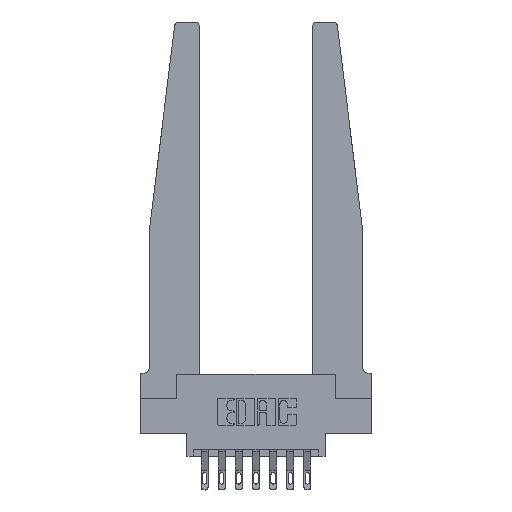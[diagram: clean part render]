
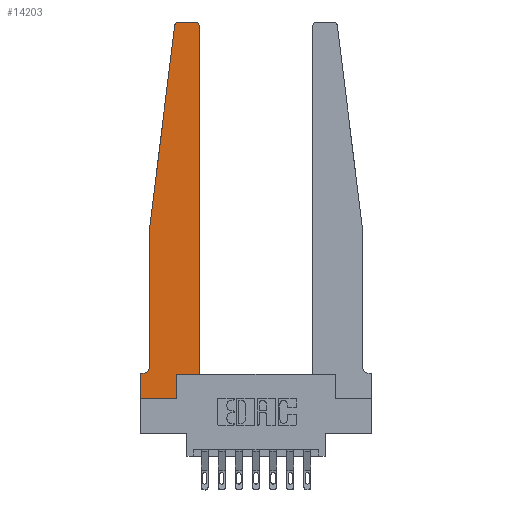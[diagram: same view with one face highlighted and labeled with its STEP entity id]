
A CAD part, top view. The second image highlights one B-rep face of the part: STEP entity #14203.
In plain terms, the highlighted planar face has unit normal (0, 0, 1).
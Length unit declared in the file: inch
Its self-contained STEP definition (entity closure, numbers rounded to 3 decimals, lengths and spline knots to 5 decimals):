
#32 = VECTOR ( 'NONE', #11932, 39.37008 ) ;
#229 = VERTEX_POINT ( 'NONE', #10092 ) ;
#743 = DIRECTION ( 'NONE',  ( 1., 0., 0. ) ) ;
#828 = ORIENTED_EDGE ( 'NONE', *, *, #6885, .T. ) ;
#1132 = LINE ( 'NONE', #3993, #10768 ) ;
#1146 = CARTESIAN_POINT ( 'NONE',  ( 0.425, 0.18, 0.37 ) ) ;
#1162 = LINE ( 'NONE', #5644, #12735 ) ;
#1504 = AXIS2_PLACEMENT_3D ( 'NONE', #10184, #3507, #11305 ) ;
#1545 = CIRCLE ( 'NONE', #8567, 0.03 ) ;
#1856 = CARTESIAN_POINT ( 'NONE',  ( 0.065, 1.25, 0.37 ) ) ;
#2055 = CIRCLE ( 'NONE', #1504, 0.03 ) ;
#2508 = CARTESIAN_POINT ( 'NONE',  ( 0.2605, 0.18, 0.37 ) ) ;
#2769 = ORIENTED_EDGE ( 'NONE', *, *, #12678, .T. ) ;
#2907 = VERTEX_POINT ( 'NONE', #9553 ) ;
#3063 = LINE ( 'NONE', #1856, #32 ) ;
#3101 = VERTEX_POINT ( 'NONE', #4327 ) ;
#3221 = DIRECTION ( 'NONE',  ( 0., 0., -1. ) ) ;
#3439 = LINE ( 'NONE', #7762, #12011 ) ;
#3442 = VERTEX_POINT ( 'NONE', #4909 ) ;
#3507 = DIRECTION ( 'NONE',  ( 0., 0., 1. ) ) ;
#3847 = VERTEX_POINT ( 'NONE', #13353 ) ;
#3967 = VERTEX_POINT ( 'NONE', #5984 ) ;
#3993 = CARTESIAN_POINT ( 'NONE',  ( 0.065, 0.1875, 0.37 ) ) ;
#4327 = CARTESIAN_POINT ( 'NONE',  ( 0.395, 2.75, 0.37 ) ) ;
#4518 = DIRECTION ( 'NONE',  ( 1., 0., 0. ) ) ;
#4674 = ORIENTED_EDGE ( 'NONE', *, *, #8214, .T. ) ;
#4909 = CARTESIAN_POINT ( 'NONE',  ( 0.015, 0.1875, 0.37 ) ) ;
#4940 = CARTESIAN_POINT ( 'NONE',  ( 0.25, 2.75, 0.37 ) ) ;
#4961 = EDGE_CURVE ( 'NONE', #229, #10171, #3439, .T. ) ;
#5064 = CARTESIAN_POINT ( 'NONE',  ( 0., 0., 0.37 ) ) ;
#5192 = EDGE_CURVE ( 'NONE', #8469, #3847, #1162, .T. ) ;
#5567 = VECTOR ( 'NONE', #12802, 39.37008 ) ;
#5644 = CARTESIAN_POINT ( 'NONE',  ( 0.425, 0.18, 0.37 ) ) ;
#5746 = EDGE_LOOP ( 'NONE', ( #14242, #11404, #11060, #9795, #4674, #6761, #11561, #2769, #8191, #8168, #828, #10840 ) ) ;
#5984 = CARTESIAN_POINT ( 'NONE',  ( 0.065, 1.25, 0.37 ) ) ;
#6089 = DIRECTION ( 'NONE',  ( 0., -1., 0. ) ) ;
#6100 = CARTESIAN_POINT ( 'NONE',  ( 0.27653, 2.75, 0.37 ) ) ;
#6177 = EDGE_CURVE ( 'NONE', #3442, #229, #1132, .T. ) ;
#6191 = AXIS2_PLACEMENT_3D ( 'NONE', #12996, #7507, #743 ) ;
#6268 = CARTESIAN_POINT ( 'NONE',  ( 0.065, 0.2375, 0.37 ) ) ;
#6617 = CARTESIAN_POINT ( 'NONE',  ( 0.395, 2.72, 0.37 ) ) ;
#6739 = VECTOR ( 'NONE', #6089, 39.37008 ) ;
#6761 = ORIENTED_EDGE ( 'NONE', *, *, #6177, .T. ) ;
#6885 = EDGE_CURVE ( 'NONE', #3847, #11098, #13203, .T. ) ;
#7171 = EDGE_CURVE ( 'NONE', #3967, #11634, #9698, .T. ) ;
#7303 = DIRECTION ( 'NONE',  ( 1., 0., 0. ) ) ;
#7507 = DIRECTION ( 'NONE',  ( 0., 0., 1. ) ) ;
#7746 = DIRECTION ( 'NONE',  ( 1., 0., 0. ) ) ;
#7762 = CARTESIAN_POINT ( 'NONE',  ( 0., 0., 0.37 ) ) ;
#7849 = DIRECTION ( 'NONE',  ( 0., 1., 0. ) ) ;
#7981 = VECTOR ( 'NONE', #7849, 39.37008 ) ;
#8168 = ORIENTED_EDGE ( 'NONE', *, *, #5192, .T. ) ;
#8180 = VECTOR ( 'NONE', #13836, 39.37008 ) ;
#8191 = ORIENTED_EDGE ( 'NONE', *, *, #10972, .T. ) ;
#8214 = EDGE_CURVE ( 'NONE', #11634, #3442, #13986, .T. ) ;
#8331 = CARTESIAN_POINT ( 'NONE',  ( 0.065, 1.25, 0.37 ) ) ;
#8426 = CARTESIAN_POINT ( 'NONE',  ( 0.2605, 0.18, 0.37 ) ) ;
#8469 = VERTEX_POINT ( 'NONE', #2508 ) ;
#8567 = AXIS2_PLACEMENT_3D ( 'NONE', #6617, #14389, #7746 ) ;
#8788 = CARTESIAN_POINT ( 'NONE',  ( 0.24675, 2.72367, 0.37 ) ) ;
#8820 = FACE_OUTER_BOUND ( 'NONE', #5746, .T. ) ;
#9223 = LINE ( 'NONE', #5064, #11796 ) ;
#9236 = CARTESIAN_POINT ( 'NONE',  ( 0., 0., 0.37 ) ) ;
#9553 = CARTESIAN_POINT ( 'NONE',  ( 0.2605, 0., 0.37 ) ) ;
#9601 = EDGE_CURVE ( 'NONE', #11098, #3101, #1545, .T. ) ;
#9698 = LINE ( 'NONE', #8331, #6739 ) ;
#9761 = EDGE_CURVE ( 'NONE', #12636, #12319, #2055, .T. ) ;
#9795 = ORIENTED_EDGE ( 'NONE', *, *, #7171, .T. ) ;
#9897 = CARTESIAN_POINT ( 'NONE',  ( 0.015, 0.2375, 0.37 ) ) ;
#10092 = CARTESIAN_POINT ( 'NONE',  ( 0., 0.1875, 0.37 ) ) ;
#10171 = VERTEX_POINT ( 'NONE', #9236 ) ;
#10184 = CARTESIAN_POINT ( 'NONE',  ( 0.27653, 2.72, 0.37 ) ) ;
#10768 = VECTOR ( 'NONE', #11779, 39.37008 ) ;
#10833 = CARTESIAN_POINT ( 'NONE',  ( 0.425, 2.72, 0.37 ) ) ;
#10840 = ORIENTED_EDGE ( 'NONE', *, *, #9601, .T. ) ;
#10972 = EDGE_CURVE ( 'NONE', #2907, #8469, #14449, .T. ) ;
#11020 = DIRECTION ( 'NONE',  ( -1., 0., 0. ) ) ;
#11060 = ORIENTED_EDGE ( 'NONE', *, *, #12209, .T. ) ;
#11098 = VERTEX_POINT ( 'NONE', #10833 ) ;
#11106 = LINE ( 'NONE', #4940, #8180 ) ;
#11305 = DIRECTION ( 'NONE',  ( 1., 0., 0. ) ) ;
#11404 = ORIENTED_EDGE ( 'NONE', *, *, #9761, .T. ) ;
#11481 = EDGE_CURVE ( 'NONE', #3101, #12636, #11106, .T. ) ;
#11561 = ORIENTED_EDGE ( 'NONE', *, *, #4961, .T. ) ;
#11634 = VERTEX_POINT ( 'NONE', #6268 ) ;
#11779 = DIRECTION ( 'NONE',  ( -1., 0., 0. ) ) ;
#11796 = VECTOR ( 'NONE', #7303, 39.37008 ) ;
#11932 = DIRECTION ( 'NONE',  ( -0.122, -0.992, 0. ) ) ;
#12011 = VECTOR ( 'NONE', #13288, 39.37008 ) ;
#12209 = EDGE_CURVE ( 'NONE', #12319, #3967, #3063, .T. ) ;
#12319 = VERTEX_POINT ( 'NONE', #8788 ) ;
#12636 = VERTEX_POINT ( 'NONE', #6100 ) ;
#12678 = EDGE_CURVE ( 'NONE', #10171, #2907, #9223, .T. ) ;
#12735 = VECTOR ( 'NONE', #4518, 39.37008 ) ;
#12802 = DIRECTION ( 'NONE',  ( 0., 1., 0. ) ) ;
#12996 = CARTESIAN_POINT ( 'NONE',  ( 0., 0.1875, 0.37 ) ) ;
#13203 = LINE ( 'NONE', #1146, #7981 ) ;
#13288 = DIRECTION ( 'NONE',  ( 0., -1., 0. ) ) ;
#13353 = CARTESIAN_POINT ( 'NONE',  ( 0.425, 0.18, 0.37 ) ) ;
#13378 = AXIS2_PLACEMENT_3D ( 'NONE', #9897, #3221, #11020 ) ;
#13836 = DIRECTION ( 'NONE',  ( -1., 0., 0. ) ) ;
#13986 = CIRCLE ( 'NONE', #13378, 0.05 ) ;
#14156 = PLANE ( 'NONE',  #6191 ) ;
#14203 = ADVANCED_FACE ( 'NONE', ( #8820 ), #14156, .T. ) ;
#14242 = ORIENTED_EDGE ( 'NONE', *, *, #11481, .T. ) ;
#14389 = DIRECTION ( 'NONE',  ( 0., 0., 1. ) ) ;
#14449 = LINE ( 'NONE', #8426, #5567 ) ;
